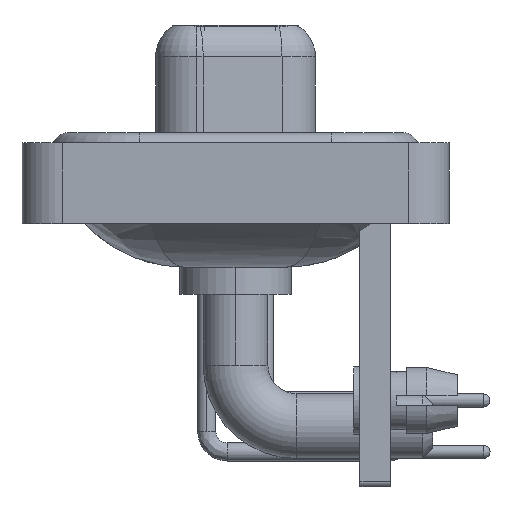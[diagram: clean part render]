
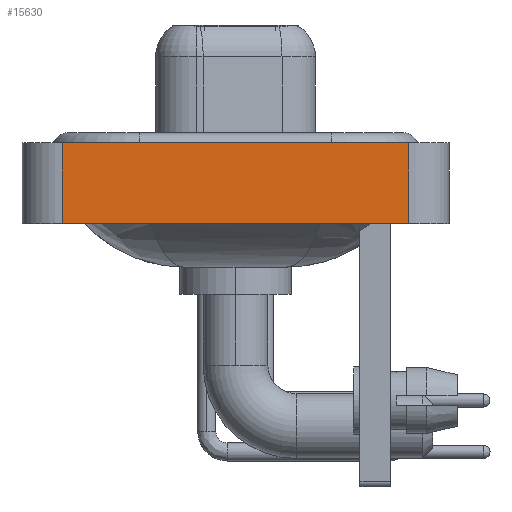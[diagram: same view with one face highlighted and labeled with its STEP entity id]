
A CAD part, left-side view. The second image highlights one B-rep face of the part: STEP entity #15630.
In plain terms, the highlighted planar face has unit normal (-1, 0, 0).
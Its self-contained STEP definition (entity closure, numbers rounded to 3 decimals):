
#407 = FACE_OUTER_BOUND ( 'NONE', #3523, .T. ) ;
#496 = DIRECTION ( 'NONE',  ( 0., -1., 0. ) ) ;
#649 = VECTOR ( 'NONE', #496, 1000. ) ;
#1039 = CARTESIAN_POINT ( 'NONE',  ( -7.35, 8.55, -3.6 ) ) ;
#3249 = CARTESIAN_POINT ( 'NONE',  ( -7.35, -8.55, 0.4 ) ) ;
#3523 = EDGE_LOOP ( 'NONE', ( #17912, #7551, #15247, #9494 ) ) ;
#3581 = VERTEX_POINT ( 'NONE', #8332 ) ;
#3625 = CARTESIAN_POINT ( 'NONE',  ( -7.35, 8.55, -3.6 ) ) ;
#4220 = PLANE ( 'NONE',  #21023 ) ;
#4228 = VECTOR ( 'NONE', #6470, 1000. ) ;
#4333 = DIRECTION ( 'NONE',  ( -1., 0., 0. ) ) ;
#6470 = DIRECTION ( 'NONE',  ( 0., -1., 0. ) ) ;
#6881 = EDGE_CURVE ( 'NONE', #20067, #15598, #19929, .T. ) ;
#7449 = VERTEX_POINT ( 'NONE', #16462 ) ;
#7551 = ORIENTED_EDGE ( 'NONE', *, *, #21132, .F. ) ;
#8332 = CARTESIAN_POINT ( 'NONE',  ( -7.35, -8.55, 0.4 ) ) ;
#8574 = LINE ( 'NONE', #3249, #4228 ) ;
#9325 = DIRECTION ( 'NONE',  ( 0., 0., 1. ) ) ;
#9444 = CARTESIAN_POINT ( 'NONE',  ( -7.35, 8.55, 0.4 ) ) ;
#9494 = ORIENTED_EDGE ( 'NONE', *, *, #10338, .T. ) ;
#10338 = EDGE_CURVE ( 'NONE', #20067, #7449, #16199, .T. ) ;
#10579 = LINE ( 'NONE', #17719, #12537 ) ;
#12537 = VECTOR ( 'NONE', #19988, 1000. ) ;
#14787 = DIRECTION ( 'NONE',  ( 0., 0., 1. ) ) ;
#15247 = ORIENTED_EDGE ( 'NONE', *, *, #6881, .F. ) ;
#15598 = VERTEX_POINT ( 'NONE', #9444 ) ;
#15630 = ADVANCED_FACE ( 'NONE', ( #407 ), #4220, .T. ) ;
#16199 = LINE ( 'NONE', #23464, #649 ) ;
#16462 = CARTESIAN_POINT ( 'NONE',  ( -7.35, -8.55, -3.6 ) ) ;
#17719 = CARTESIAN_POINT ( 'NONE',  ( -7.35, -8.55, -3.6 ) ) ;
#17912 = ORIENTED_EDGE ( 'NONE', *, *, #21584, .T. ) ;
#18479 = VECTOR ( 'NONE', #14787, 1000. ) ;
#19929 = LINE ( 'NONE', #3625, #18479 ) ;
#19988 = DIRECTION ( 'NONE',  ( 0., 0., 1. ) ) ;
#20067 = VERTEX_POINT ( 'NONE', #1039 ) ;
#21023 = AXIS2_PLACEMENT_3D ( 'NONE', #22419, #4333, #9325 ) ;
#21132 = EDGE_CURVE ( 'NONE', #15598, #3581, #8574, .T. ) ;
#21584 = EDGE_CURVE ( 'NONE', #7449, #3581, #10579, .T. ) ;
#22419 = CARTESIAN_POINT ( 'NONE',  ( -7.35, -8.55, -3.6 ) ) ;
#23464 = CARTESIAN_POINT ( 'NONE',  ( -7.35, -8.55, -3.6 ) ) ;
